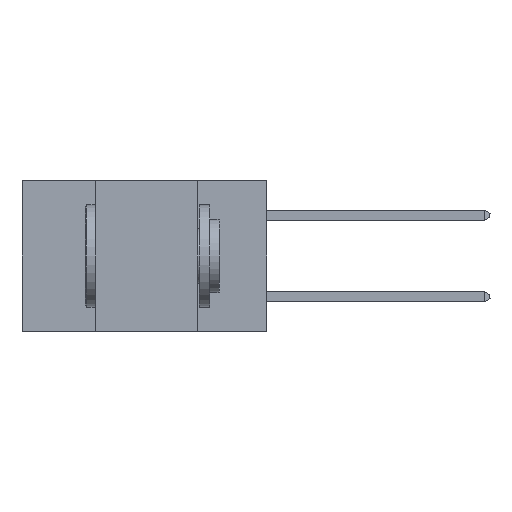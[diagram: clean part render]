
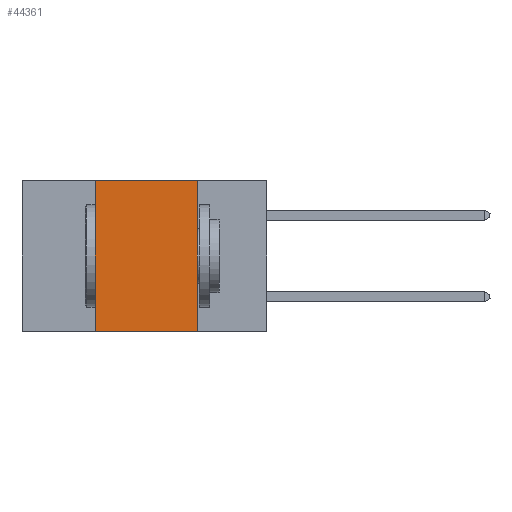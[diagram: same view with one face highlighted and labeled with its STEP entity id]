
A CAD part, left-side view. The second image highlights one B-rep face of the part: STEP entity #44361.
In plain terms, the highlighted planar face has unit normal (-1, 0, 0).
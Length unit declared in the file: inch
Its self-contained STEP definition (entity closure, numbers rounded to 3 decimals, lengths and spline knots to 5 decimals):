
#553 = DIRECTION ( 'NONE',  ( 1., 0., 0. ) ) ;
#2276 = ORIENTED_EDGE ( 'NONE', *, *, #25905, .F. ) ;
#8788 = EDGE_CURVE ( 'NONE', #22680, #27983, #38522, .T. ) ;
#9585 = LINE ( 'NONE', #39900, #36040 ) ;
#9668 = CARTESIAN_POINT ( 'NONE',  ( 0., 0.17, -0.37 ) ) ;
#9746 = DIRECTION ( 'NONE',  ( 0., 0., 1. ) ) ;
#9792 = LINE ( 'NONE', #18314, #22158 ) ;
#10850 = CARTESIAN_POINT ( 'NONE',  ( 0., 0.6, 0. ) ) ;
#12114 = LINE ( 'NONE', #39091, #20553 ) ;
#14206 = DIRECTION ( 'NONE',  ( 0., 0., -1. ) ) ;
#14305 = CARTESIAN_POINT ( 'NONE',  ( 0., 0.42, 0. ) ) ;
#18314 = CARTESIAN_POINT ( 'NONE',  ( 0., 0.6, -0.37 ) ) ;
#20553 = VECTOR ( 'NONE', #24739, 39.37008 ) ;
#21690 = CARTESIAN_POINT ( 'NONE',  ( 0., 0.17, 0. ) ) ;
#22158 = VECTOR ( 'NONE', #43550, 39.37008 ) ;
#22168 = DIRECTION ( 'NONE',  ( 0., 0., -1. ) ) ;
#22680 = VERTEX_POINT ( 'NONE', #45700 ) ;
#23286 = VECTOR ( 'NONE', #9746, 39.37008 ) ;
#24739 = DIRECTION ( 'NONE',  ( 0., -1., 0. ) ) ;
#25905 = EDGE_CURVE ( 'NONE', #27983, #26825, #12114, .T. ) ;
#26825 = VERTEX_POINT ( 'NONE', #21690 ) ;
#27983 = VERTEX_POINT ( 'NONE', #14305 ) ;
#29424 = ORIENTED_EDGE ( 'NONE', *, *, #43551, .F. ) ;
#30821 = EDGE_LOOP ( 'NONE', ( #29424, #2276, #44923, #36737 ) ) ;
#31295 = CARTESIAN_POINT ( 'NONE',  ( 0., 0.42, 0. ) ) ;
#33719 = FACE_OUTER_BOUND ( 'NONE', #30821, .T. ) ;
#34687 = EDGE_CURVE ( 'NONE', #22680, #38957, #9792, .T. ) ;
#36040 = VECTOR ( 'NONE', #14206, 39.37008 ) ;
#36737 = ORIENTED_EDGE ( 'NONE', *, *, #34687, .T. ) ;
#38522 = LINE ( 'NONE', #31295, #23286 ) ;
#38957 = VERTEX_POINT ( 'NONE', #9668 ) ;
#39002 = AXIS2_PLACEMENT_3D ( 'NONE', #10850, #553, #22168 ) ;
#39091 = CARTESIAN_POINT ( 'NONE',  ( 0., 0.6, 0. ) ) ;
#39900 = CARTESIAN_POINT ( 'NONE',  ( 0., 0.17, 0. ) ) ;
#43550 = DIRECTION ( 'NONE',  ( 0., -1., 0. ) ) ;
#43551 = EDGE_CURVE ( 'NONE', #26825, #38957, #9585, .T. ) ;
#43807 = PLANE ( 'NONE',  #39002 ) ;
#44361 = ADVANCED_FACE ( 'NONE', ( #33719 ), #43807, .F. ) ;
#44923 = ORIENTED_EDGE ( 'NONE', *, *, #8788, .F. ) ;
#45700 = CARTESIAN_POINT ( 'NONE',  ( 0., 0.42, -0.37 ) ) ;
